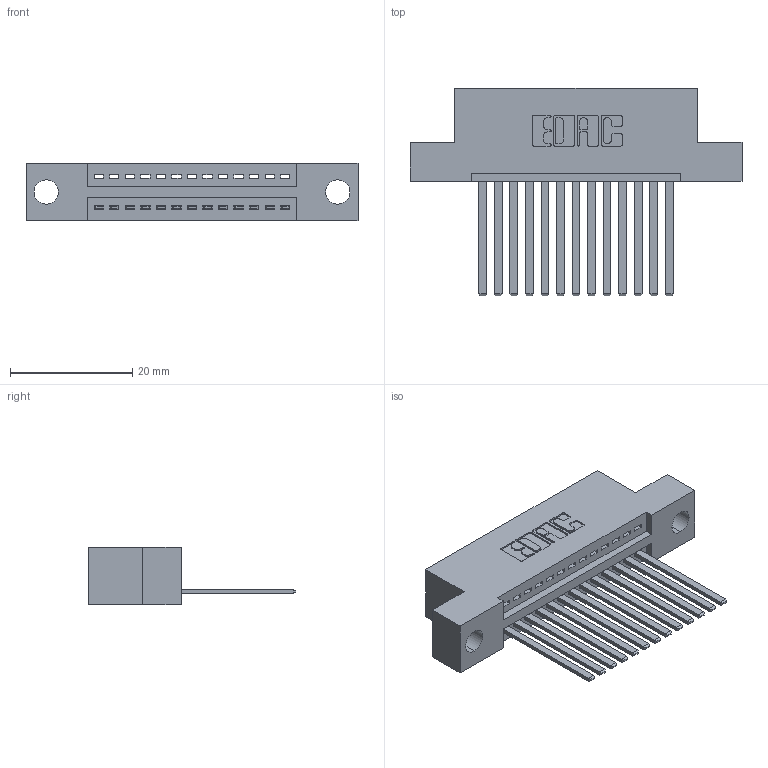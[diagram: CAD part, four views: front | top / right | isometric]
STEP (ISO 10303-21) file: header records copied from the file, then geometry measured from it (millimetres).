
FILE_DESCRIPTION (( 'STEP AP203' ), '1' );
FILE_NAME ('345-013-544-104.STEP', '2021-05-26T14:10:55', ( '' ), ( '' ), 'SwSTEP 2.0', 'SolidWorks 2020', '' );
FILE_SCHEMA (( 'CONFIG_CONTROL_DESIGN' ));
Length unit declared in the file: inch
Products named in the file (3): 345-013-544-104; 345 Part_Flush Mounting Lugs - 0.156 Dia-TI; 345-292-001_345-293-144
Assembly tree (14 placements, depth 2):
  345-013-544-104
    345 Part_Flush Mounting Lugs - 0.156 Dia-TI
    345-292-001_345-293-144  x13
Bounding box: 54.23 x 33.96 x 9.4 mm (x, y, z)
Volume: 4957.8 mm3; surface area: 6488.8 mm2
Topology: 14 solids, 14 shells, 816 faces, 2431 edges, 1602 vertices
Faces by surface type: plane 562, cylinder 254
Entity records: 13923 total; most frequent: CARTESIAN_POINT 2421, ORIENTED_EDGE 2366, DIRECTION 2153, EDGE_CURVE 1183, LINE 1003, VECTOR 1003, VERTEX_POINT 786, AXIS2_PLACEMENT_3D 575
